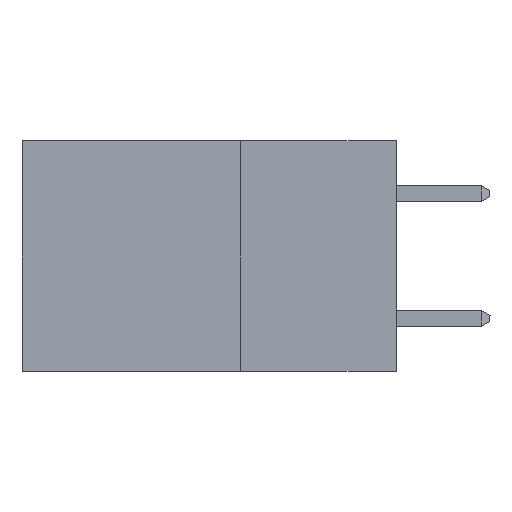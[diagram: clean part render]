
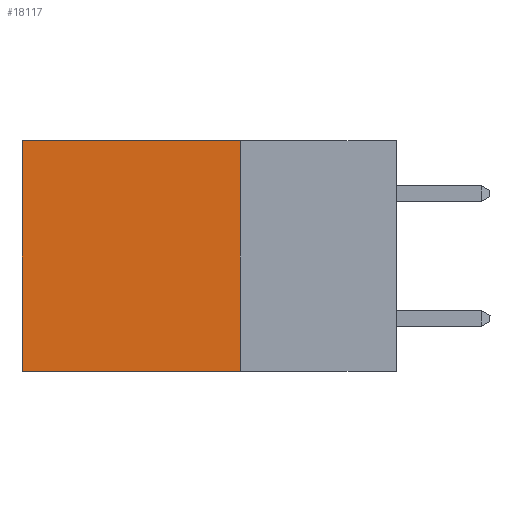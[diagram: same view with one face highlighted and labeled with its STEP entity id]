
A CAD part, left-side view. The second image highlights one B-rep face of the part: STEP entity #18117.
In plain terms, the highlighted planar face has unit normal (-1, 0, 0).
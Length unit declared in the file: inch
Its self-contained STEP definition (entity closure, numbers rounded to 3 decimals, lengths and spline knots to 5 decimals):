
#44 = EDGE_CURVE ( 'NONE', #2559, #17063, #3976, .T. ) ;
#502 = VECTOR ( 'NONE', #3979, 39.37008 ) ;
#1096 = EDGE_LOOP ( 'NONE', ( #12147, #11914, #16723, #4957 ) ) ;
#1588 = VECTOR ( 'NONE', #3762, 39.37008 ) ;
#2559 = VERTEX_POINT ( 'NONE', #11437 ) ;
#2911 = FACE_OUTER_BOUND ( 'NONE', #1096, .T. ) ;
#3762 = DIRECTION ( 'NONE',  ( 0., 1., 0. ) ) ;
#3858 = CARTESIAN_POINT ( 'NONE',  ( 0.2615, 0.6, -0.37 ) ) ;
#3976 = LINE ( 'NONE', #3858, #502 ) ;
#3979 = DIRECTION ( 'NONE',  ( 0., 0., -1. ) ) ;
#4713 = LINE ( 'NONE', #12399, #11842 ) ;
#4957 = ORIENTED_EDGE ( 'NONE', *, *, #16268, .T. ) ;
#5477 = CARTESIAN_POINT ( 'NONE',  ( 0.2615, 0.25, -0.37 ) ) ;
#6913 = DIRECTION ( 'NONE',  ( 1., 0., 0. ) ) ;
#7787 = CARTESIAN_POINT ( 'NONE',  ( 0.2615, 0.25, 0. ) ) ;
#7981 = AXIS2_PLACEMENT_3D ( 'NONE', #5477, #6913, #16821 ) ;
#8804 = CARTESIAN_POINT ( 'NONE',  ( 0.2615, 0.25, -0.37 ) ) ;
#9643 = VERTEX_POINT ( 'NONE', #10568 ) ;
#10568 = CARTESIAN_POINT ( 'NONE',  ( 0.2615, 0.25, -0.37 ) ) ;
#11437 = CARTESIAN_POINT ( 'NONE',  ( 0.2615, 0.6, 0. ) ) ;
#11842 = VECTOR ( 'NONE', #13849, 39.37008 ) ;
#11914 = ORIENTED_EDGE ( 'NONE', *, *, #18001, .F. ) ;
#12147 = ORIENTED_EDGE ( 'NONE', *, *, #44, .T. ) ;
#12399 = CARTESIAN_POINT ( 'NONE',  ( 0.2615, 0.25, -0.37 ) ) ;
#13156 = DIRECTION ( 'NONE',  ( 0., 0., -1. ) ) ;
#13178 = VECTOR ( 'NONE', #13156, 39.37008 ) ;
#13627 = LINE ( 'NONE', #8804, #13178 ) ;
#13725 = CARTESIAN_POINT ( 'NONE',  ( 0.2615, 0.25, 0. ) ) ;
#13849 = DIRECTION ( 'NONE',  ( 0., 1., 0. ) ) ;
#14028 = PLANE ( 'NONE',  #7981 ) ;
#14149 = VERTEX_POINT ( 'NONE', #7787 ) ;
#15886 = CARTESIAN_POINT ( 'NONE',  ( 0.2615, 0.6, -0.37 ) ) ;
#16268 = EDGE_CURVE ( 'NONE', #14149, #2559, #16286, .T. ) ;
#16286 = LINE ( 'NONE', #13725, #1588 ) ;
#16723 = ORIENTED_EDGE ( 'NONE', *, *, #18370, .F. ) ;
#16821 = DIRECTION ( 'NONE',  ( 0., 0., -1. ) ) ;
#17063 = VERTEX_POINT ( 'NONE', #15886 ) ;
#18001 = EDGE_CURVE ( 'NONE', #9643, #17063, #4713, .T. ) ;
#18117 = ADVANCED_FACE ( 'NONE', ( #2911 ), #14028, .F. ) ;
#18370 = EDGE_CURVE ( 'NONE', #14149, #9643, #13627, .T. ) ;
